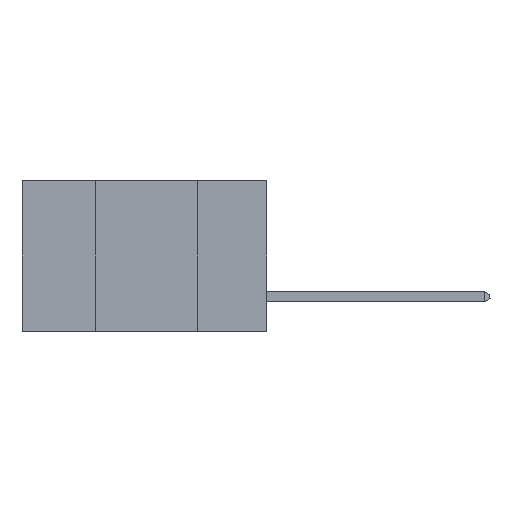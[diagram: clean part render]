
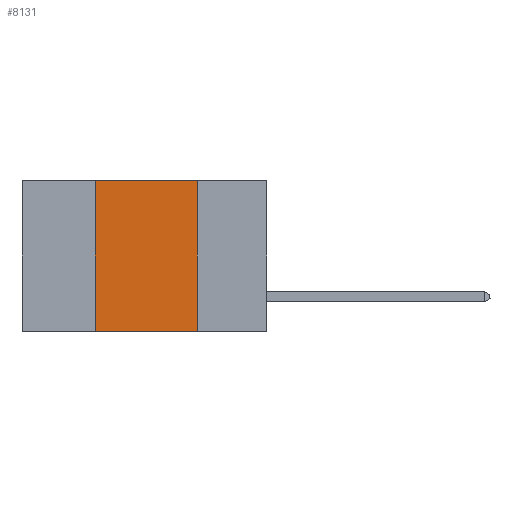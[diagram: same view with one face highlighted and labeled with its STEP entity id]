
A CAD part, left-side view. The second image highlights one B-rep face of the part: STEP entity #8131.
In plain terms, the highlighted planar face has unit normal (-1, 0, 0).
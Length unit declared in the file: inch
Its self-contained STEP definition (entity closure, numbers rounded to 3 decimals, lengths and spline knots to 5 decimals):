
#184 = LINE ( 'NONE', #8057, #4119 ) ;
#231 = CARTESIAN_POINT ( 'NONE',  ( 0., 0.17, -0.37 ) ) ;
#428 = DIRECTION ( 'NONE',  ( 0., 0., -1. ) ) ;
#483 = VECTOR ( 'NONE', #518, 39.37008 ) ;
#518 = DIRECTION ( 'NONE',  ( 0., 0., 1. ) ) ;
#607 = EDGE_LOOP ( 'NONE', ( #3648, #6937, #1135, #1809 ) ) ;
#1135 = ORIENTED_EDGE ( 'NONE', *, *, #6608, .F. ) ;
#1187 = VERTEX_POINT ( 'NONE', #231 ) ;
#1343 = LINE ( 'NONE', #3175, #3020 ) ;
#1809 = ORIENTED_EDGE ( 'NONE', *, *, #2761, .T. ) ;
#2356 = DIRECTION ( 'NONE',  ( 0., 0., -1. ) ) ;
#2489 = DIRECTION ( 'NONE',  ( 0., -1., 0. ) ) ;
#2761 = EDGE_CURVE ( 'NONE', #8562, #1187, #12155, .T. ) ;
#3020 = VECTOR ( 'NONE', #4156, 39.37008 ) ;
#3175 = CARTESIAN_POINT ( 'NONE',  ( 0., 0.6, 0. ) ) ;
#3648 = ORIENTED_EDGE ( 'NONE', *, *, #6320, .F. ) ;
#3906 = CARTESIAN_POINT ( 'NONE',  ( 0., 0.6, 0. ) ) ;
#4119 = VECTOR ( 'NONE', #2356, 39.37008 ) ;
#4156 = DIRECTION ( 'NONE',  ( 0., -1., 0. ) ) ;
#4744 = PLANE ( 'NONE',  #12135 ) ;
#5632 = VECTOR ( 'NONE', #2489, 39.37008 ) ;
#6320 = EDGE_CURVE ( 'NONE', #9254, #1187, #184, .T. ) ;
#6608 = EDGE_CURVE ( 'NONE', #8562, #10456, #7020, .T. ) ;
#6937 = ORIENTED_EDGE ( 'NONE', *, *, #9931, .F. ) ;
#7020 = LINE ( 'NONE', #9311, #483 ) ;
#7043 = CARTESIAN_POINT ( 'NONE',  ( 0., 0.42, -0.37 ) ) ;
#8057 = CARTESIAN_POINT ( 'NONE',  ( 0., 0.17, 0. ) ) ;
#8131 = ADVANCED_FACE ( 'NONE', ( #11594 ), #4744, .F. ) ;
#8317 = DIRECTION ( 'NONE',  ( 1., 0., 0. ) ) ;
#8334 = CARTESIAN_POINT ( 'NONE',  ( 0., 0.6, -0.37 ) ) ;
#8562 = VERTEX_POINT ( 'NONE', #7043 ) ;
#9062 = CARTESIAN_POINT ( 'NONE',  ( 0., 0.42, 0. ) ) ;
#9254 = VERTEX_POINT ( 'NONE', #9963 ) ;
#9311 = CARTESIAN_POINT ( 'NONE',  ( 0., 0.42, 0. ) ) ;
#9931 = EDGE_CURVE ( 'NONE', #10456, #9254, #1343, .T. ) ;
#9963 = CARTESIAN_POINT ( 'NONE',  ( 0., 0.17, 0. ) ) ;
#10456 = VERTEX_POINT ( 'NONE', #9062 ) ;
#11594 = FACE_OUTER_BOUND ( 'NONE', #607, .T. ) ;
#12135 = AXIS2_PLACEMENT_3D ( 'NONE', #3906, #8317, #428 ) ;
#12155 = LINE ( 'NONE', #8334, #5632 ) ;
